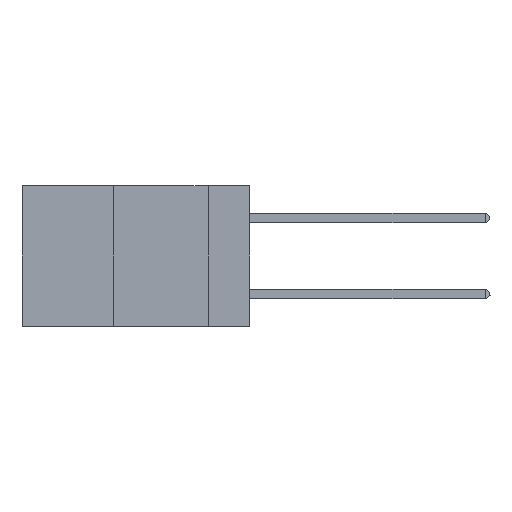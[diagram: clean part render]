
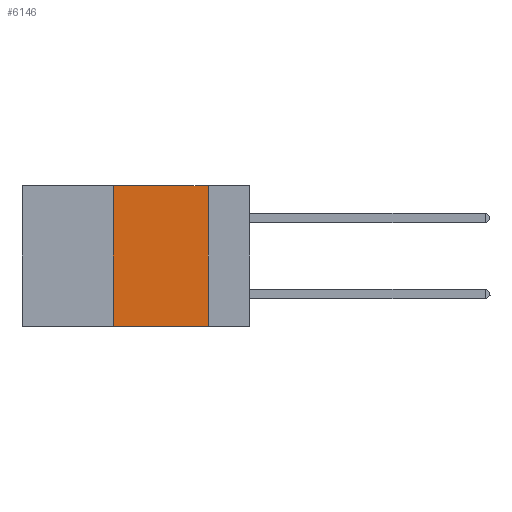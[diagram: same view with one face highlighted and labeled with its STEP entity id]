
A CAD part, left-side view. The second image highlights one B-rep face of the part: STEP entity #6146.
In plain terms, the highlighted planar face has unit normal (-1, 0, 0).
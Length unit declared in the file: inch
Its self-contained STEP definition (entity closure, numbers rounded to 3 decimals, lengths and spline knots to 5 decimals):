
#565 = ORIENTED_EDGE ( 'NONE', *, *, #16617, .F. ) ;
#938 = DIRECTION ( 'NONE',  ( 0., 0., -1. ) ) ;
#1980 = DIRECTION ( 'NONE',  ( 0., 0., 1. ) ) ;
#2529 = LINE ( 'NONE', #5211, #12422 ) ;
#2729 = EDGE_CURVE ( 'NONE', #11796, #5826, #8701, .T. ) ;
#5211 = CARTESIAN_POINT ( 'NONE',  ( 0., 0.36, 0. ) ) ;
#5783 = ORIENTED_EDGE ( 'NONE', *, *, #2729, .F. ) ;
#5826 = VERTEX_POINT ( 'NONE', #18195 ) ;
#6146 = ADVANCED_FACE ( 'NONE', ( #9480 ), #10372, .F. ) ;
#6186 = CARTESIAN_POINT ( 'NONE',  ( 0., 0.6, 0. ) ) ;
#6393 = AXIS2_PLACEMENT_3D ( 'NONE', #12075, #13793, #938 ) ;
#6710 = EDGE_CURVE ( 'NONE', #15962, #5826, #11402, .T. ) ;
#8023 = ORIENTED_EDGE ( 'NONE', *, *, #6710, .T. ) ;
#8079 = DIRECTION ( 'NONE',  ( 0., -1., 0. ) ) ;
#8402 = EDGE_LOOP ( 'NONE', ( #5783, #17198, #565, #8023 ) ) ;
#8701 = LINE ( 'NONE', #11361, #16380 ) ;
#9162 = EDGE_CURVE ( 'NONE', #12677, #11796, #18291, .T. ) ;
#9480 = FACE_OUTER_BOUND ( 'NONE', #8402, .T. ) ;
#10166 = VECTOR ( 'NONE', #13299, 39.37008 ) ;
#10372 = PLANE ( 'NONE',  #6393 ) ;
#11361 = CARTESIAN_POINT ( 'NONE',  ( 0., 0.11, 0. ) ) ;
#11402 = LINE ( 'NONE', #13514, #10166 ) ;
#11796 = VERTEX_POINT ( 'NONE', #17017 ) ;
#12075 = CARTESIAN_POINT ( 'NONE',  ( 0., 0.6, 0. ) ) ;
#12354 = CARTESIAN_POINT ( 'NONE',  ( 0., 0.36, -0.37 ) ) ;
#12422 = VECTOR ( 'NONE', #1980, 39.37008 ) ;
#12677 = VERTEX_POINT ( 'NONE', #16899 ) ;
#13299 = DIRECTION ( 'NONE',  ( 0., -1., 0. ) ) ;
#13514 = CARTESIAN_POINT ( 'NONE',  ( 0., 0.6, -0.37 ) ) ;
#13793 = DIRECTION ( 'NONE',  ( 1., 0., 0. ) ) ;
#14052 = VECTOR ( 'NONE', #8079, 39.37008 ) ;
#14528 = DIRECTION ( 'NONE',  ( 0., 0., -1. ) ) ;
#15962 = VERTEX_POINT ( 'NONE', #12354 ) ;
#16380 = VECTOR ( 'NONE', #14528, 39.37008 ) ;
#16617 = EDGE_CURVE ( 'NONE', #15962, #12677, #2529, .T. ) ;
#16899 = CARTESIAN_POINT ( 'NONE',  ( 0., 0.36, 0. ) ) ;
#17017 = CARTESIAN_POINT ( 'NONE',  ( 0., 0.11, 0. ) ) ;
#17198 = ORIENTED_EDGE ( 'NONE', *, *, #9162, .F. ) ;
#18195 = CARTESIAN_POINT ( 'NONE',  ( 0., 0.11, -0.37 ) ) ;
#18291 = LINE ( 'NONE', #6186, #14052 ) ;
